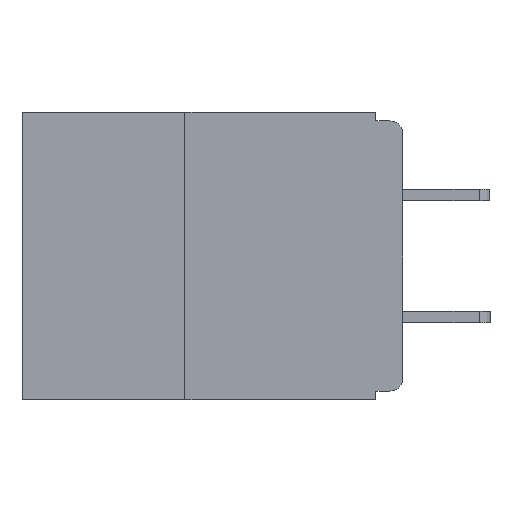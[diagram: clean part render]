
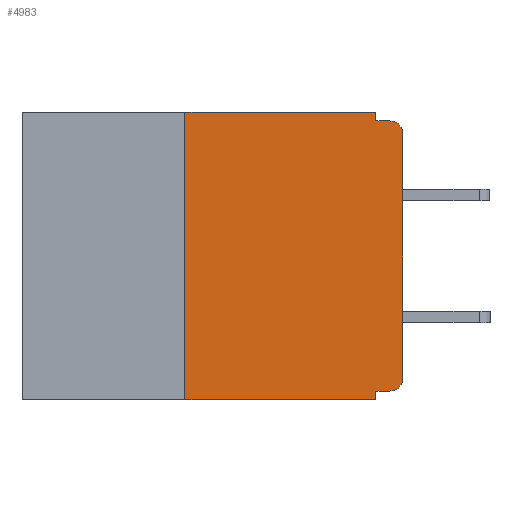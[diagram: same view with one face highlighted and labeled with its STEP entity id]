
A CAD part, left-side view. The second image highlights one B-rep face of the part: STEP entity #4983.
In plain terms, the highlighted planar face has unit normal (-1, 0, 0).
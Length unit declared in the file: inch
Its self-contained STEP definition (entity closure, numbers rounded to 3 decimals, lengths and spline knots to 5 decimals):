
#46 = VECTOR ( 'NONE', #14094, 39.37008 ) ;
#166 = CARTESIAN_POINT ( 'NONE',  ( 0., 0.25, -0.33 ) ) ;
#280 = CARTESIAN_POINT ( 'NONE',  ( 0., 0.031, -0.32 ) ) ;
#416 = CARTESIAN_POINT ( 'NONE',  ( 0., 0., -0.305 ) ) ;
#663 = EDGE_CURVE ( 'NONE', #9701, #6935, #11125, .T. ) ;
#762 = LINE ( 'NONE', #13687, #10329 ) ;
#844 = VERTEX_POINT ( 'NONE', #166 ) ;
#1191 = VECTOR ( 'NONE', #12185, 39.37008 ) ;
#1275 = ORIENTED_EDGE ( 'NONE', *, *, #12191, .T. ) ;
#1318 = ORIENTED_EDGE ( 'NONE', *, *, #3229, .F. ) ;
#1600 = CARTESIAN_POINT ( 'NONE',  ( 0., 0.25, -0.33 ) ) ;
#1642 = VERTEX_POINT ( 'NONE', #416 ) ;
#1769 = VERTEX_POINT ( 'NONE', #11944 ) ;
#1798 = ORIENTED_EDGE ( 'NONE', *, *, #10810, .F. ) ;
#1827 = VERTEX_POINT ( 'NONE', #12332 ) ;
#1844 = ORIENTED_EDGE ( 'NONE', *, *, #11104, .F. ) ;
#2056 = LINE ( 'NONE', #13825, #5940 ) ;
#2348 = ORIENTED_EDGE ( 'NONE', *, *, #8819, .F. ) ;
#2895 = CARTESIAN_POINT ( 'NONE',  ( 0., 0.015, -0.305 ) ) ;
#2909 = VERTEX_POINT ( 'NONE', #4900 ) ;
#2934 = ORIENTED_EDGE ( 'NONE', *, *, #663, .T. ) ;
#3122 = ORIENTED_EDGE ( 'NONE', *, *, #12555, .T. ) ;
#3229 = EDGE_CURVE ( 'NONE', #844, #9409, #11773, .T. ) ;
#4252 = LINE ( 'NONE', #14137, #46 ) ;
#4443 = EDGE_CURVE ( 'NONE', #2909, #1642, #13864, .T. ) ;
#4778 = AXIS2_PLACEMENT_3D ( 'NONE', #8853, #8805, #10515 ) ;
#4900 = CARTESIAN_POINT ( 'NONE',  ( 0., 0.015, -0.32 ) ) ;
#4907 = DIRECTION ( 'NONE',  ( -1., 0., 0. ) ) ;
#4983 = ADVANCED_FACE ( 'NONE', ( #11717 ), #15391, .F. ) ;
#5211 = VECTOR ( 'NONE', #6902, 39.37008 ) ;
#5518 = DIRECTION ( 'NONE',  ( 0., 1., 0. ) ) ;
#5838 = DIRECTION ( 'NONE',  ( 0., -1., 0. ) ) ;
#5940 = VECTOR ( 'NONE', #5518, 39.37008 ) ;
#6902 = DIRECTION ( 'NONE',  ( 0., -1., 0. ) ) ;
#6935 = VERTEX_POINT ( 'NONE', #14344 ) ;
#7707 = EDGE_LOOP ( 'NONE', ( #3122, #2934, #2348, #1844, #1798, #1318, #1275, #8885, #8908, #8821 ) ) ;
#7786 = VECTOR ( 'NONE', #8971, 39.37008 ) ;
#8160 = CARTESIAN_POINT ( 'NONE',  ( 0., 0.437, 0. ) ) ;
#8805 = DIRECTION ( 'NONE',  ( -1., 0., 0. ) ) ;
#8819 = EDGE_CURVE ( 'NONE', #11880, #6935, #762, .T. ) ;
#8821 = ORIENTED_EDGE ( 'NONE', *, *, #4443, .T. ) ;
#8853 = CARTESIAN_POINT ( 'NONE',  ( 0., 0.015, -0.025 ) ) ;
#8885 = ORIENTED_EDGE ( 'NONE', *, *, #9453, .F. ) ;
#8908 = ORIENTED_EDGE ( 'NONE', *, *, #13758, .F. ) ;
#8971 = DIRECTION ( 'NONE',  ( 0., 0., 1. ) ) ;
#9409 = VERTEX_POINT ( 'NONE', #14679 ) ;
#9453 = EDGE_CURVE ( 'NONE', #13142, #1769, #4252, .T. ) ;
#9701 = VERTEX_POINT ( 'NONE', #11514 ) ;
#9809 = LINE ( 'NONE', #15227, #12881 ) ;
#10110 = CARTESIAN_POINT ( 'NONE',  ( 0., 0., 0. ) ) ;
#10329 = VECTOR ( 'NONE', #13519, 39.37008 ) ;
#10515 = DIRECTION ( 'NONE',  ( 0., 0., -1. ) ) ;
#10810 = EDGE_CURVE ( 'NONE', #9409, #1827, #14683, .T. ) ;
#11048 = DIRECTION ( 'NONE',  ( 0., 0., -1. ) ) ;
#11104 = EDGE_CURVE ( 'NONE', #1827, #11880, #14128, .T. ) ;
#11125 = CIRCLE ( 'NONE', #4778, 0.015 ) ;
#11208 = CARTESIAN_POINT ( 'NONE',  ( 0., 0.031, -0.01 ) ) ;
#11242 = LINE ( 'NONE', #10110, #7786 ) ;
#11514 = CARTESIAN_POINT ( 'NONE',  ( 0., 0., -0.025 ) ) ;
#11717 = FACE_OUTER_BOUND ( 'NONE', #7707, .T. ) ;
#11773 = LINE ( 'NONE', #1600, #14424 ) ;
#11880 = VERTEX_POINT ( 'NONE', #11208 ) ;
#11944 = CARTESIAN_POINT ( 'NONE',  ( 0., 0.031, -0.33 ) ) ;
#12185 = DIRECTION ( 'NONE',  ( 0., 0., -1. ) ) ;
#12191 = EDGE_CURVE ( 'NONE', #844, #1769, #9809, .T. ) ;
#12332 = CARTESIAN_POINT ( 'NONE',  ( 0., 0.031, 0. ) ) ;
#12509 = AXIS2_PLACEMENT_3D ( 'NONE', #2895, #4907, #11048 ) ;
#12555 = EDGE_CURVE ( 'NONE', #1642, #9701, #11242, .T. ) ;
#12881 = VECTOR ( 'NONE', #5838, 39.37008 ) ;
#13142 = VERTEX_POINT ( 'NONE', #280 ) ;
#13519 = DIRECTION ( 'NONE',  ( 0., -1., 0. ) ) ;
#13687 = CARTESIAN_POINT ( 'NONE',  ( 0., 0., -0.01 ) ) ;
#13758 = EDGE_CURVE ( 'NONE', #2909, #13142, #2056, .T. ) ;
#13825 = CARTESIAN_POINT ( 'NONE',  ( 0., 0., -0.32 ) ) ;
#13864 = CIRCLE ( 'NONE', #12509, 0.015 ) ;
#14094 = DIRECTION ( 'NONE',  ( 0., 0., -1. ) ) ;
#14128 = LINE ( 'NONE', #15547, #1191 ) ;
#14137 = CARTESIAN_POINT ( 'NONE',  ( 0., 0.031, -0.33 ) ) ;
#14344 = CARTESIAN_POINT ( 'NONE',  ( 0., 0.015, -0.01 ) ) ;
#14424 = VECTOR ( 'NONE', #15687, 39.37008 ) ;
#14679 = CARTESIAN_POINT ( 'NONE',  ( 0., 0.25, 0. ) ) ;
#14683 = LINE ( 'NONE', #8160, #5211 ) ;
#14963 = AXIS2_PLACEMENT_3D ( 'NONE', #15376, #15346, #15322 ) ;
#15227 = CARTESIAN_POINT ( 'NONE',  ( 0., 0.437, -0.33 ) ) ;
#15322 = DIRECTION ( 'NONE',  ( 0., 0., -1. ) ) ;
#15346 = DIRECTION ( 'NONE',  ( 1., 0., 0. ) ) ;
#15376 = CARTESIAN_POINT ( 'NONE',  ( 0., 0.437, 0. ) ) ;
#15391 = PLANE ( 'NONE',  #14963 ) ;
#15547 = CARTESIAN_POINT ( 'NONE',  ( 0., 0.031, 0. ) ) ;
#15687 = DIRECTION ( 'NONE',  ( 0., 0., 1. ) ) ;
